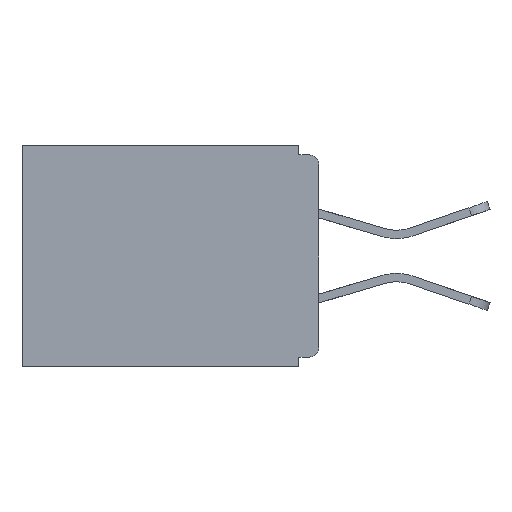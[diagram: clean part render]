
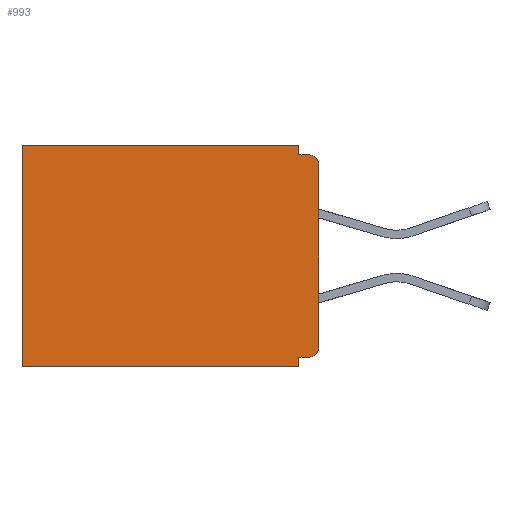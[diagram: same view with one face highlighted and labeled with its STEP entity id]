
A CAD part, left-side view. The second image highlights one B-rep face of the part: STEP entity #993.
In plain terms, the highlighted planar face has unit normal (-1, 0, 0).
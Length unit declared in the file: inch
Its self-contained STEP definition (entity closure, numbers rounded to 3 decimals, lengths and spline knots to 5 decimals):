
#34 = EDGE_CURVE ( 'NONE', #17731, #15425, #9479, .T. ) ;
#87 = DIRECTION ( 'NONE',  ( 0., -1., 0. ) ) ;
#375 = CARTESIAN_POINT ( 'NONE',  ( 0.298, 0.031, -0.328 ) ) ;
#555 = LINE ( 'NONE', #19212, #19028 ) ;
#573 = CARTESIAN_POINT ( 'NONE',  ( 0.298, 0., -0.03 ) ) ;
#630 = CARTESIAN_POINT ( 'NONE',  ( 0.298, 0., 0. ) ) ;
#695 = ORIENTED_EDGE ( 'NONE', *, *, #17540, .F. ) ;
#822 = VECTOR ( 'NONE', #5171, 39.37008 ) ;
#902 = DIRECTION ( 'NONE',  ( 0., 0., -1. ) ) ;
#910 = VECTOR ( 'NONE', #87, 39.37008 ) ;
#942 = CARTESIAN_POINT ( 'NONE',  ( 0.298, 0., -0.343 ) ) ;
#993 = ADVANCED_FACE ( 'NONE', ( #13785 ), #14655, .F. ) ;
#1410 = VECTOR ( 'NONE', #6795, 39.37008 ) ;
#1640 = CARTESIAN_POINT ( 'NONE',  ( 0.298, 0., -0.015 ) ) ;
#1864 = AXIS2_PLACEMENT_3D ( 'NONE', #19334, #5429, #902 ) ;
#1996 = LINE ( 'NONE', #19081, #13757 ) ;
#2425 = DIRECTION ( 'NONE',  ( 0., 0., -1. ) ) ;
#2462 = LINE ( 'NONE', #6834, #7001 ) ;
#2484 = CARTESIAN_POINT ( 'NONE',  ( 0.298, 0.015, -0.328 ) ) ;
#2519 = EDGE_CURVE ( 'NONE', #17051, #2765, #8684, .T. ) ;
#2765 = VERTEX_POINT ( 'NONE', #6035 ) ;
#3245 = LINE ( 'NONE', #630, #14014 ) ;
#3597 = CARTESIAN_POINT ( 'NONE',  ( 0.298, 0.46, 0. ) ) ;
#3843 = ORIENTED_EDGE ( 'NONE', *, *, #7457, .T. ) ;
#3864 = CARTESIAN_POINT ( 'NONE',  ( 0.298, 0.015, -0.03 ) ) ;
#4195 = EDGE_CURVE ( 'NONE', #12574, #16677, #5300, .T. ) ;
#4267 = EDGE_LOOP ( 'NONE', ( #9291, #12322, #13971, #3843, #12657, #16810, #695, #17949, #4312, #15099 ) ) ;
#4312 = ORIENTED_EDGE ( 'NONE', *, *, #2519, .T. ) ;
#4496 = LINE ( 'NONE', #1640, #910 ) ;
#5171 = DIRECTION ( 'NONE',  ( 0., 1., 0. ) ) ;
#5300 = CIRCLE ( 'NONE', #13142, 0.015 ) ;
#5429 = DIRECTION ( 'NONE',  ( 1., 0., 0. ) ) ;
#5489 = CARTESIAN_POINT ( 'NONE',  ( 0.298, 0.031, -0.343 ) ) ;
#5688 = DIRECTION ( 'NONE',  ( -1., 0., 0. ) ) ;
#6035 = CARTESIAN_POINT ( 'NONE',  ( 0.298, 0., -0.313 ) ) ;
#6300 = CARTESIAN_POINT ( 'NONE',  ( 0.298, 0.031, 0. ) ) ;
#6767 = CARTESIAN_POINT ( 'NONE',  ( 0.298, 0., -0.328 ) ) ;
#6795 = DIRECTION ( 'NONE',  ( 0., 0., -1. ) ) ;
#6805 = LINE ( 'NONE', #942, #14481 ) ;
#6834 = CARTESIAN_POINT ( 'NONE',  ( 0.298, 0., 0. ) ) ;
#6856 = DIRECTION ( 'NONE',  ( 0., 1., 0. ) ) ;
#7001 = VECTOR ( 'NONE', #2425, 39.37008 ) ;
#7457 = EDGE_CURVE ( 'NONE', #19326, #17731, #3245, .T. ) ;
#8398 = VERTEX_POINT ( 'NONE', #15892 ) ;
#8684 = CIRCLE ( 'NONE', #19786, 0.015 ) ;
#9291 = ORIENTED_EDGE ( 'NONE', *, *, #4195, .T. ) ;
#9479 = LINE ( 'NONE', #3597, #1410 ) ;
#9697 = DIRECTION ( 'NONE',  ( 0., 1., 0. ) ) ;
#9956 = CARTESIAN_POINT ( 'NONE',  ( 0.298, 0.015, -0.313 ) ) ;
#10012 = CARTESIAN_POINT ( 'NONE',  ( 0.298, 0.46, -0.343 ) ) ;
#10532 = EDGE_CURVE ( 'NONE', #8398, #16677, #4496, .T. ) ;
#11322 = DIRECTION ( 'NONE',  ( 0., 0., -1. ) ) ;
#11557 = DIRECTION ( 'NONE',  ( -1., 0., 0. ) ) ;
#11581 = VERTEX_POINT ( 'NONE', #5489 ) ;
#11949 = CARTESIAN_POINT ( 'NONE',  ( 0.298, 0.46, 0. ) ) ;
#12032 = EDGE_CURVE ( 'NONE', #11581, #15425, #6805, .T. ) ;
#12097 = LINE ( 'NONE', #6767, #822 ) ;
#12322 = ORIENTED_EDGE ( 'NONE', *, *, #10532, .F. ) ;
#12574 = VERTEX_POINT ( 'NONE', #573 ) ;
#12585 = EDGE_CURVE ( 'NONE', #17051, #16374, #12097, .T. ) ;
#12657 = ORIENTED_EDGE ( 'NONE', *, *, #34, .T. ) ;
#12691 = EDGE_CURVE ( 'NONE', #12574, #2765, #2462, .T. ) ;
#12935 = DIRECTION ( 'NONE',  ( 0., 0., -1. ) ) ;
#13026 = DIRECTION ( 'NONE',  ( 0., 0., -1. ) ) ;
#13142 = AXIS2_PLACEMENT_3D ( 'NONE', #3864, #5688, #12935 ) ;
#13338 = EDGE_CURVE ( 'NONE', #19326, #8398, #555, .T. ) ;
#13757 = VECTOR ( 'NONE', #11322, 39.37008 ) ;
#13785 = FACE_OUTER_BOUND ( 'NONE', #4267, .T. ) ;
#13971 = ORIENTED_EDGE ( 'NONE', *, *, #13338, .F. ) ;
#14014 = VECTOR ( 'NONE', #9697, 39.37008 ) ;
#14481 = VECTOR ( 'NONE', #6856, 39.37008 ) ;
#14655 = PLANE ( 'NONE',  #1864 ) ;
#15099 = ORIENTED_EDGE ( 'NONE', *, *, #12691, .F. ) ;
#15425 = VERTEX_POINT ( 'NONE', #10012 ) ;
#15892 = CARTESIAN_POINT ( 'NONE',  ( 0.298, 0.031, -0.015 ) ) ;
#16374 = VERTEX_POINT ( 'NONE', #375 ) ;
#16677 = VERTEX_POINT ( 'NONE', #19057 ) ;
#16810 = ORIENTED_EDGE ( 'NONE', *, *, #12032, .F. ) ;
#16956 = DIRECTION ( 'NONE',  ( 0., 0., -1. ) ) ;
#17051 = VERTEX_POINT ( 'NONE', #2484 ) ;
#17540 = EDGE_CURVE ( 'NONE', #16374, #11581, #1996, .T. ) ;
#17731 = VERTEX_POINT ( 'NONE', #11949 ) ;
#17949 = ORIENTED_EDGE ( 'NONE', *, *, #12585, .F. ) ;
#19028 = VECTOR ( 'NONE', #16956, 39.37008 ) ;
#19057 = CARTESIAN_POINT ( 'NONE',  ( 0.298, 0.015, -0.015 ) ) ;
#19081 = CARTESIAN_POINT ( 'NONE',  ( 0.298, 0.031, -0.343 ) ) ;
#19212 = CARTESIAN_POINT ( 'NONE',  ( 0.298, 0.031, -0.343 ) ) ;
#19326 = VERTEX_POINT ( 'NONE', #6300 ) ;
#19334 = CARTESIAN_POINT ( 'NONE',  ( 0.298, 0., 0. ) ) ;
#19786 = AXIS2_PLACEMENT_3D ( 'NONE', #9956, #11557, #13026 ) ;
